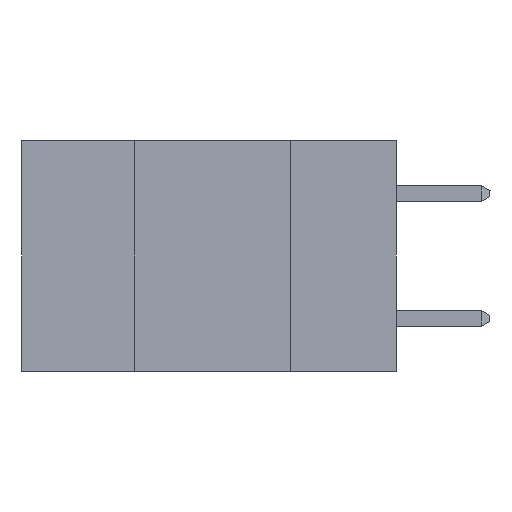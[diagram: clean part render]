
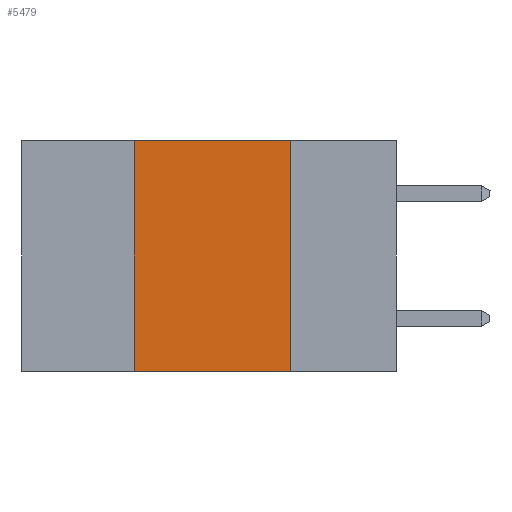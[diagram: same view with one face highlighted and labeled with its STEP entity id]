
A CAD part, left-side view. The second image highlights one B-rep face of the part: STEP entity #5479.
In plain terms, the highlighted planar face has unit normal (-1, 0, 0).
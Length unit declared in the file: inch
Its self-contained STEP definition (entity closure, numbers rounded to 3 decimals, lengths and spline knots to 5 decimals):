
#90 = CARTESIAN_POINT ( 'NONE',  ( 0., 0.42, -0.37 ) ) ;
#421 = EDGE_CURVE ( 'NONE', #4887, #7229, #1130, .T. ) ;
#688 = EDGE_CURVE ( 'NONE', #6178, #6428, #5693, .T. ) ;
#1130 = LINE ( 'NONE', #9929, #10221 ) ;
#2225 = FACE_OUTER_BOUND ( 'NONE', #2555, .T. ) ;
#2555 = EDGE_LOOP ( 'NONE', ( #7791, #5473, #3101, #9850 ) ) ;
#2970 = VECTOR ( 'NONE', #6480, 39.37008 ) ;
#3101 = ORIENTED_EDGE ( 'NONE', *, *, #8932, .F. ) ;
#3184 = CARTESIAN_POINT ( 'NONE',  ( 0., 0.17, -0.37 ) ) ;
#3766 = DIRECTION ( 'NONE',  ( 0., 0., -1. ) ) ;
#3819 = CARTESIAN_POINT ( 'NONE',  ( 0., 0.42, 0. ) ) ;
#4176 = DIRECTION ( 'NONE',  ( 0., 0., -1. ) ) ;
#4539 = DIRECTION ( 'NONE',  ( 1., 0., 0. ) ) ;
#4647 = PLANE ( 'NONE',  #6906 ) ;
#4887 = VERTEX_POINT ( 'NONE', #7297 ) ;
#5360 = LINE ( 'NONE', #3819, #2970 ) ;
#5473 = ORIENTED_EDGE ( 'NONE', *, *, #421, .F. ) ;
#5479 = ADVANCED_FACE ( 'NONE', ( #2225 ), #4647, .F. ) ;
#5693 = LINE ( 'NONE', #10267, #6236 ) ;
#6178 = VERTEX_POINT ( 'NONE', #90 ) ;
#6236 = VECTOR ( 'NONE', #9359, 39.37008 ) ;
#6245 = EDGE_CURVE ( 'NONE', #7229, #6428, #10709, .T. ) ;
#6312 = VECTOR ( 'NONE', #3766, 39.37008 ) ;
#6428 = VERTEX_POINT ( 'NONE', #3184 ) ;
#6480 = DIRECTION ( 'NONE',  ( 0., 0., 1. ) ) ;
#6906 = AXIS2_PLACEMENT_3D ( 'NONE', #9715, #4539, #4176 ) ;
#7229 = VERTEX_POINT ( 'NONE', #7807 ) ;
#7297 = CARTESIAN_POINT ( 'NONE',  ( 0., 0.42, 0. ) ) ;
#7791 = ORIENTED_EDGE ( 'NONE', *, *, #6245, .F. ) ;
#7807 = CARTESIAN_POINT ( 'NONE',  ( 0., 0.17, 0. ) ) ;
#8932 = EDGE_CURVE ( 'NONE', #6178, #4887, #5360, .T. ) ;
#9080 = CARTESIAN_POINT ( 'NONE',  ( 0., 0.17, 0. ) ) ;
#9359 = DIRECTION ( 'NONE',  ( 0., -1., 0. ) ) ;
#9715 = CARTESIAN_POINT ( 'NONE',  ( 0., 0.6, 0. ) ) ;
#9777 = DIRECTION ( 'NONE',  ( 0., -1., 0. ) ) ;
#9850 = ORIENTED_EDGE ( 'NONE', *, *, #688, .T. ) ;
#9929 = CARTESIAN_POINT ( 'NONE',  ( 0., 0.6, 0. ) ) ;
#10221 = VECTOR ( 'NONE', #9777, 39.37008 ) ;
#10267 = CARTESIAN_POINT ( 'NONE',  ( 0., 0.6, -0.37 ) ) ;
#10709 = LINE ( 'NONE', #9080, #6312 ) ;
